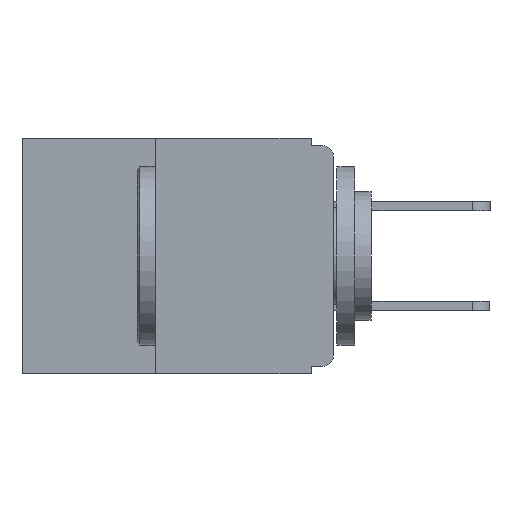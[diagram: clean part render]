
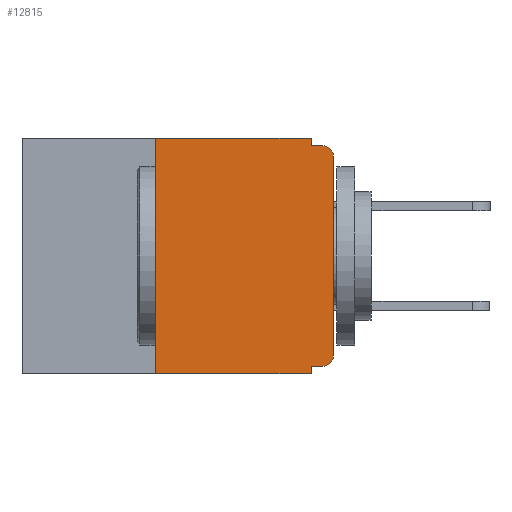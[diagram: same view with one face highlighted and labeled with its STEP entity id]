
A CAD part, left-side view. The second image highlights one B-rep face of the part: STEP entity #12815.
In plain terms, the highlighted planar face has unit normal (-1, 0, 0).
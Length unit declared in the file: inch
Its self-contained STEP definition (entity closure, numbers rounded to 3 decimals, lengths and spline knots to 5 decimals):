
#87 = VECTOR ( 'NONE', #8758, 39.37008 ) ;
#184 = VERTEX_POINT ( 'NONE', #13310 ) ;
#252 = DIRECTION ( 'NONE',  ( 0., 0., -1. ) ) ;
#348 = VERTEX_POINT ( 'NONE', #4057 ) ;
#635 = DIRECTION ( 'NONE',  ( -1., 0., 0. ) ) ;
#781 = EDGE_CURVE ( 'NONE', #12969, #6122, #1412, .T. ) ;
#956 = AXIS2_PLACEMENT_3D ( 'NONE', #3748, #13599, #7044 ) ;
#1077 = DIRECTION ( 'NONE',  ( 0., 0., -1. ) ) ;
#1122 = FACE_OUTER_BOUND ( 'NONE', #11534, .T. ) ;
#1211 = CARTESIAN_POINT ( 'NONE',  ( 0., 0.031, -0.32 ) ) ;
#1257 = CARTESIAN_POINT ( 'NONE',  ( 0., 0., 0. ) ) ;
#1306 = VERTEX_POINT ( 'NONE', #9338 ) ;
#1412 = LINE ( 'NONE', #9140, #11694 ) ;
#1533 = LINE ( 'NONE', #9959, #9960 ) ;
#1710 = ORIENTED_EDGE ( 'NONE', *, *, #10762, .T. ) ;
#1797 = CARTESIAN_POINT ( 'NONE',  ( 0., 0., -0.32 ) ) ;
#1813 = CARTESIAN_POINT ( 'NONE',  ( 0., 0.015, -0.32 ) ) ;
#2050 = CIRCLE ( 'NONE', #6098, 0.015 ) ;
#2112 = VECTOR ( 'NONE', #11339, 39.37008 ) ;
#2265 = EDGE_CURVE ( 'NONE', #5902, #184, #1533, .T. ) ;
#2383 = LINE ( 'NONE', #9221, #13678 ) ;
#2777 = LINE ( 'NONE', #1257, #5356 ) ;
#2919 = EDGE_CURVE ( 'NONE', #184, #12969, #2383, .T. ) ;
#3088 = LINE ( 'NONE', #5438, #87 ) ;
#3210 = CARTESIAN_POINT ( 'NONE',  ( 0., 0.015, -0.01 ) ) ;
#3326 = ORIENTED_EDGE ( 'NONE', *, *, #9851, .T. ) ;
#3577 = EDGE_CURVE ( 'NONE', #5931, #4770, #5986, .T. ) ;
#3748 = CARTESIAN_POINT ( 'NONE',  ( 0., 0.437, 0. ) ) ;
#4030 = EDGE_CURVE ( 'NONE', #5902, #1306, #3088, .T. ) ;
#4057 = CARTESIAN_POINT ( 'NONE',  ( 0., 0., -0.025 ) ) ;
#4757 = EDGE_CURVE ( 'NONE', #4770, #1306, #14155, .T. ) ;
#4770 = VERTEX_POINT ( 'NONE', #1211 ) ;
#4788 = CARTESIAN_POINT ( 'NONE',  ( 0., 0., -0.01 ) ) ;
#4966 = ORIENTED_EDGE ( 'NONE', *, *, #8244, .T. ) ;
#5142 = CARTESIAN_POINT ( 'NONE',  ( 0., 0.031, 0. ) ) ;
#5356 = VECTOR ( 'NONE', #10052, 39.37008 ) ;
#5397 = ORIENTED_EDGE ( 'NONE', *, *, #3577, .F. ) ;
#5438 = CARTESIAN_POINT ( 'NONE',  ( 0., 0.437, -0.33 ) ) ;
#5513 = CARTESIAN_POINT ( 'NONE',  ( 0., 0.25, -0.33 ) ) ;
#5768 = ORIENTED_EDGE ( 'NONE', *, *, #7443, .F. ) ;
#5902 = VERTEX_POINT ( 'NONE', #5513 ) ;
#5931 = VERTEX_POINT ( 'NONE', #1813 ) ;
#5986 = LINE ( 'NONE', #1797, #11448 ) ;
#6098 = AXIS2_PLACEMENT_3D ( 'NONE', #7230, #635, #8326 ) ;
#6122 = VERTEX_POINT ( 'NONE', #11013 ) ;
#6426 = VERTEX_POINT ( 'NONE', #12570 ) ;
#6864 = DIRECTION ( 'NONE',  ( -1., 0., 0. ) ) ;
#7044 = DIRECTION ( 'NONE',  ( 0., 0., -1. ) ) ;
#7230 = CARTESIAN_POINT ( 'NONE',  ( 0., 0.015, -0.305 ) ) ;
#7443 = EDGE_CURVE ( 'NONE', #6122, #11434, #7608, .T. ) ;
#7608 = LINE ( 'NONE', #4788, #2112 ) ;
#7788 = CARTESIAN_POINT ( 'NONE',  ( 0., 0.031, -0.33 ) ) ;
#8244 = EDGE_CURVE ( 'NONE', #348, #11434, #10143, .T. ) ;
#8265 = ORIENTED_EDGE ( 'NONE', *, *, #4030, .T. ) ;
#8326 = DIRECTION ( 'NONE',  ( 0., 0., -1. ) ) ;
#8656 = AXIS2_PLACEMENT_3D ( 'NONE', #13400, #6864, #252 ) ;
#8758 = DIRECTION ( 'NONE',  ( 0., -1., 0. ) ) ;
#8884 = DIRECTION ( 'NONE',  ( 0., 0., -1. ) ) ;
#9056 = DIRECTION ( 'NONE',  ( 0., -1., 0. ) ) ;
#9140 = CARTESIAN_POINT ( 'NONE',  ( 0., 0.031, 0. ) ) ;
#9221 = CARTESIAN_POINT ( 'NONE',  ( 0., 0.437, 0. ) ) ;
#9338 = CARTESIAN_POINT ( 'NONE',  ( 0., 0.031, -0.33 ) ) ;
#9537 = ORIENTED_EDGE ( 'NONE', *, *, #781, .F. ) ;
#9851 = EDGE_CURVE ( 'NONE', #6426, #348, #2777, .T. ) ;
#9959 = CARTESIAN_POINT ( 'NONE',  ( 0., 0.25, -0.33 ) ) ;
#9960 = VECTOR ( 'NONE', #10608, 39.37008 ) ;
#10052 = DIRECTION ( 'NONE',  ( 0., 0., 1. ) ) ;
#10143 = CIRCLE ( 'NONE', #8656, 0.015 ) ;
#10179 = DIRECTION ( 'NONE',  ( 0., 1., 0. ) ) ;
#10608 = DIRECTION ( 'NONE',  ( 0., 0., 1. ) ) ;
#10762 = EDGE_CURVE ( 'NONE', #5931, #6426, #2050, .T. ) ;
#11013 = CARTESIAN_POINT ( 'NONE',  ( 0., 0.031, -0.01 ) ) ;
#11339 = DIRECTION ( 'NONE',  ( 0., -1., 0. ) ) ;
#11434 = VERTEX_POINT ( 'NONE', #3210 ) ;
#11448 = VECTOR ( 'NONE', #10179, 39.37008 ) ;
#11514 = ORIENTED_EDGE ( 'NONE', *, *, #4757, .F. ) ;
#11534 = EDGE_LOOP ( 'NONE', ( #3326, #4966, #5768, #9537, #12216, #13662, #8265, #11514, #5397, #1710 ) ) ;
#11694 = VECTOR ( 'NONE', #1077, 39.37008 ) ;
#12216 = ORIENTED_EDGE ( 'NONE', *, *, #2919, .F. ) ;
#12503 = PLANE ( 'NONE',  #956 ) ;
#12570 = CARTESIAN_POINT ( 'NONE',  ( 0., 0., -0.305 ) ) ;
#12815 = ADVANCED_FACE ( 'NONE', ( #1122 ), #12503, .F. ) ;
#12969 = VERTEX_POINT ( 'NONE', #5142 ) ;
#13310 = CARTESIAN_POINT ( 'NONE',  ( 0., 0.25, 0. ) ) ;
#13400 = CARTESIAN_POINT ( 'NONE',  ( 0., 0.015, -0.025 ) ) ;
#13599 = DIRECTION ( 'NONE',  ( 1., 0., 0. ) ) ;
#13662 = ORIENTED_EDGE ( 'NONE', *, *, #2265, .F. ) ;
#13678 = VECTOR ( 'NONE', #9056, 39.37008 ) ;
#13815 = VECTOR ( 'NONE', #8884, 39.37008 ) ;
#14155 = LINE ( 'NONE', #7788, #13815 ) ;
